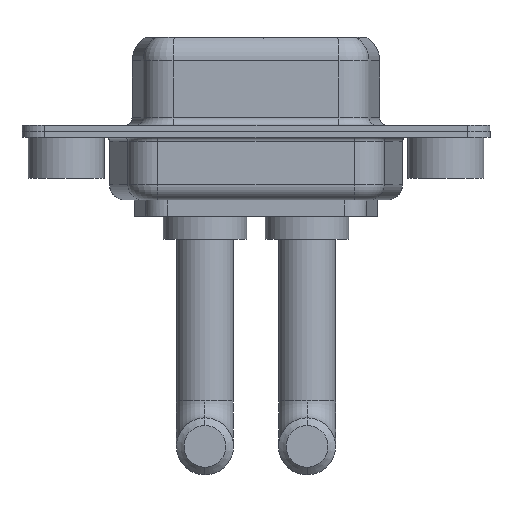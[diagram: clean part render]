
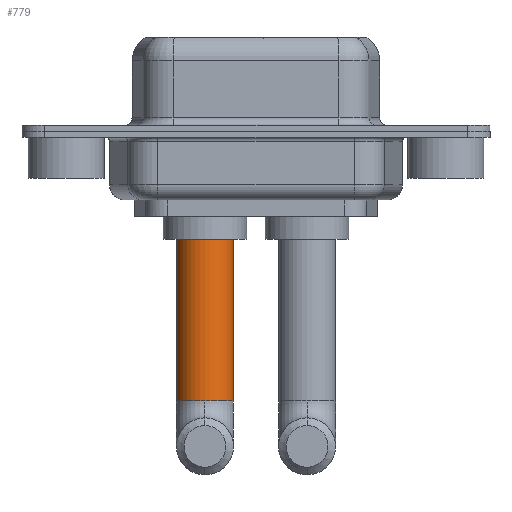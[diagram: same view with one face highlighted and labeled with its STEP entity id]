
A CAD part, front view. The second image highlights one B-rep face of the part: STEP entity #779.
In plain terms, the highlighted cylindrical face has radius 1.875 mm (diameter 3.75 mm), a partial arc.
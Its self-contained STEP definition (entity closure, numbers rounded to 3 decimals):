
#43 = VERTEX_POINT ( 'NONE', #6475 ) ;
#187 = VECTOR ( 'NONE', #9376, 1000. ) ;
#443 = CARTESIAN_POINT ( 'NONE',  ( 0., 0., -10.63 ) ) ;
#457 = CARTESIAN_POINT ( 'NONE',  ( 0., -1.875, -10.63 ) ) ;
#779 = ADVANCED_FACE ( 'NONE', ( #10448 ), #1196, .T. ) ;
#1196 = CYLINDRICAL_SURFACE ( 'NONE', #9557, 1.875 ) ;
#1551 = EDGE_CURVE ( 'NONE', #11542, #12347, #10215, .T. ) ;
#1557 = DIRECTION ( 'NONE',  ( 0., 0., -1. ) ) ;
#1651 = AXIS2_PLACEMENT_3D ( 'NONE', #443, #3249, #3508 ) ;
#3023 = CIRCLE ( 'NONE', #8617, 1.875 ) ;
#3091 = LINE ( 'NONE', #4237, #187 ) ;
#3223 = ORIENTED_EDGE ( 'NONE', *, *, #8125, .F. ) ;
#3249 = DIRECTION ( 'NONE',  ( 0., 0., -1. ) ) ;
#3333 = CARTESIAN_POINT ( 'NONE',  ( 1.875, 0., 0. ) ) ;
#3367 = EDGE_CURVE ( 'NONE', #12347, #7118, #3091, .T. ) ;
#3508 = DIRECTION ( 'NONE',  ( -1., 0., 0. ) ) ;
#3993 = VERTEX_POINT ( 'NONE', #457 ) ;
#4001 = VECTOR ( 'NONE', #5488, 1000. ) ;
#4167 = EDGE_CURVE ( 'NONE', #3993, #7118, #3023, .T. ) ;
#4237 = CARTESIAN_POINT ( 'NONE',  ( -1.875, 0., 0. ) ) ;
#4377 = AXIS2_PLACEMENT_3D ( 'NONE', #12709, #1557, #10963 ) ;
#4526 = DIRECTION ( 'NONE',  ( 0., 0., -1. ) ) ;
#4982 = CARTESIAN_POINT ( 'NONE',  ( -1.875, 0., -10.63 ) ) ;
#5084 = CIRCLE ( 'NONE', #1651, 1.875 ) ;
#5173 = DIRECTION ( 'NONE',  ( 0., 0., -1. ) ) ;
#5430 = LINE ( 'NONE', #10576, #4001 ) ;
#5488 = DIRECTION ( 'NONE',  ( 0., 0., -1. ) ) ;
#5723 = ORIENTED_EDGE ( 'NONE', *, *, #4167, .F. ) ;
#6175 = CARTESIAN_POINT ( 'NONE',  ( 0., 0., 0. ) ) ;
#6475 = CARTESIAN_POINT ( 'NONE',  ( 1.875, 0., -10.63 ) ) ;
#7118 = VERTEX_POINT ( 'NONE', #4982 ) ;
#8029 = ORIENTED_EDGE ( 'NONE', *, *, #8394, .F. ) ;
#8125 = EDGE_CURVE ( 'NONE', #11542, #43, #5430, .T. ) ;
#8349 = EDGE_LOOP ( 'NONE', ( #3223, #8659, #13087, #5723, #8029 ) ) ;
#8394 = EDGE_CURVE ( 'NONE', #43, #3993, #5084, .T. ) ;
#8617 = AXIS2_PLACEMENT_3D ( 'NONE', #10549, #4526, #10615 ) ;
#8659 = ORIENTED_EDGE ( 'NONE', *, *, #1551, .T. ) ;
#9376 = DIRECTION ( 'NONE',  ( 0., 0., -1. ) ) ;
#9557 = AXIS2_PLACEMENT_3D ( 'NONE', #6175, #5173, #11485 ) ;
#10215 = CIRCLE ( 'NONE', #4377, 1.875 ) ;
#10448 = FACE_OUTER_BOUND ( 'NONE', #8349, .T. ) ;
#10549 = CARTESIAN_POINT ( 'NONE',  ( 0., 0., -10.63 ) ) ;
#10576 = CARTESIAN_POINT ( 'NONE',  ( 1.875, 0., 0. ) ) ;
#10615 = DIRECTION ( 'NONE',  ( -1., 0., 0. ) ) ;
#10963 = DIRECTION ( 'NONE',  ( -1., 0., 0. ) ) ;
#11055 = CARTESIAN_POINT ( 'NONE',  ( -1.875, 0., 0. ) ) ;
#11485 = DIRECTION ( 'NONE',  ( -1., 0., 0. ) ) ;
#11542 = VERTEX_POINT ( 'NONE', #3333 ) ;
#12347 = VERTEX_POINT ( 'NONE', #11055 ) ;
#12709 = CARTESIAN_POINT ( 'NONE',  ( 0., 0., 0. ) ) ;
#13087 = ORIENTED_EDGE ( 'NONE', *, *, #3367, .T. ) ;
